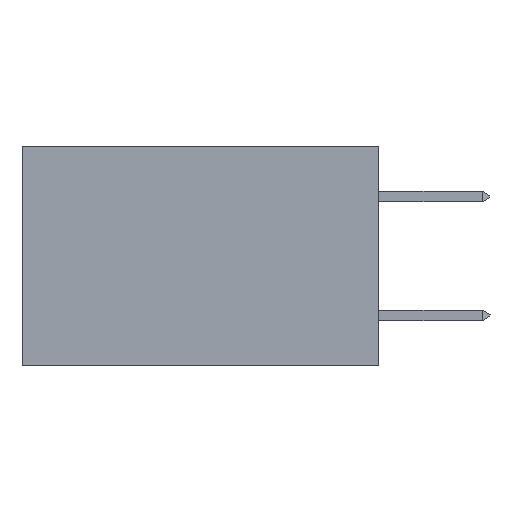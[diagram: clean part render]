
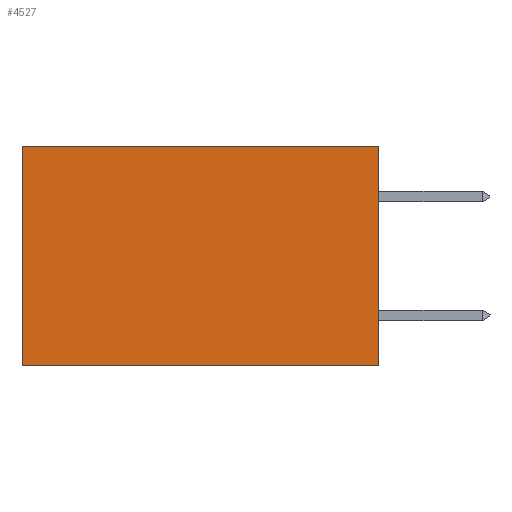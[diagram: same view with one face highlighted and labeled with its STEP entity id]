
A CAD part, left-side view. The second image highlights one B-rep face of the part: STEP entity #4527.
In plain terms, the highlighted planar face has unit normal (-1, 0, 0).
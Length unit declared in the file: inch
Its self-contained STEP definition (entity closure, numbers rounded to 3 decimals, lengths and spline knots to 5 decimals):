
#419 = EDGE_CURVE ( 'NONE', #1850, #4239, #457, .T. ) ;
#457 = LINE ( 'NONE', #15102, #16484 ) ;
#965 = VERTEX_POINT ( 'NONE', #1020 ) ;
#1020 = CARTESIAN_POINT ( 'NONE',  ( 0.298, 0.6, 0. ) ) ;
#1842 = VERTEX_POINT ( 'NONE', #15944 ) ;
#1850 = VERTEX_POINT ( 'NONE', #9920 ) ;
#3168 = EDGE_CURVE ( 'NONE', #1850, #965, #8570, .T. ) ;
#3685 = FACE_OUTER_BOUND ( 'NONE', #11426, .T. ) ;
#4164 = AXIS2_PLACEMENT_3D ( 'NONE', #11435, #8292, #19142 ) ;
#4239 = VERTEX_POINT ( 'NONE', #19100 ) ;
#4527 = ADVANCED_FACE ( 'NONE', ( #3685 ), #6728, .F. ) ;
#4849 = DIRECTION ( 'NONE',  ( 0., 1., 0. ) ) ;
#5197 = LINE ( 'NONE', #18539, #13956 ) ;
#6270 = CARTESIAN_POINT ( 'NONE',  ( 0.298, 0., 0. ) ) ;
#6728 = PLANE ( 'NONE',  #4164 ) ;
#7895 = CARTESIAN_POINT ( 'NONE',  ( 0.298, 0.6, 0. ) ) ;
#8292 = DIRECTION ( 'NONE',  ( 1., 0., 0. ) ) ;
#8570 = LINE ( 'NONE', #6270, #16059 ) ;
#8799 = ORIENTED_EDGE ( 'NONE', *, *, #16189, .T. ) ;
#9920 = CARTESIAN_POINT ( 'NONE',  ( 0.298, 0., 0. ) ) ;
#11426 = EDGE_LOOP ( 'NONE', ( #8799, #13082, #12681, #17521 ) ) ;
#11435 = CARTESIAN_POINT ( 'NONE',  ( 0.298, 0., 0. ) ) ;
#12681 = ORIENTED_EDGE ( 'NONE', *, *, #419, .F. ) ;
#13082 = ORIENTED_EDGE ( 'NONE', *, *, #16215, .F. ) ;
#13956 = VECTOR ( 'NONE', #19179, 39.37008 ) ;
#14647 = VECTOR ( 'NONE', #17733, 39.37008 ) ;
#15102 = CARTESIAN_POINT ( 'NONE',  ( 0.298, 0., 0. ) ) ;
#15944 = CARTESIAN_POINT ( 'NONE',  ( 0.298, 0.6, -0.37 ) ) ;
#16059 = VECTOR ( 'NONE', #4849, 39.37008 ) ;
#16189 = EDGE_CURVE ( 'NONE', #965, #1842, #17553, .T. ) ;
#16215 = EDGE_CURVE ( 'NONE', #4239, #1842, #5197, .T. ) ;
#16484 = VECTOR ( 'NONE', #16908, 39.37008 ) ;
#16908 = DIRECTION ( 'NONE',  ( 0., 0., -1. ) ) ;
#17521 = ORIENTED_EDGE ( 'NONE', *, *, #3168, .T. ) ;
#17553 = LINE ( 'NONE', #7895, #14647 ) ;
#17733 = DIRECTION ( 'NONE',  ( 0., 0., -1. ) ) ;
#18539 = CARTESIAN_POINT ( 'NONE',  ( 0.298, 0., -0.37 ) ) ;
#19100 = CARTESIAN_POINT ( 'NONE',  ( 0.298, 0., -0.37 ) ) ;
#19142 = DIRECTION ( 'NONE',  ( 0., 0., -1. ) ) ;
#19179 = DIRECTION ( 'NONE',  ( 0., 1., 0. ) ) ;
